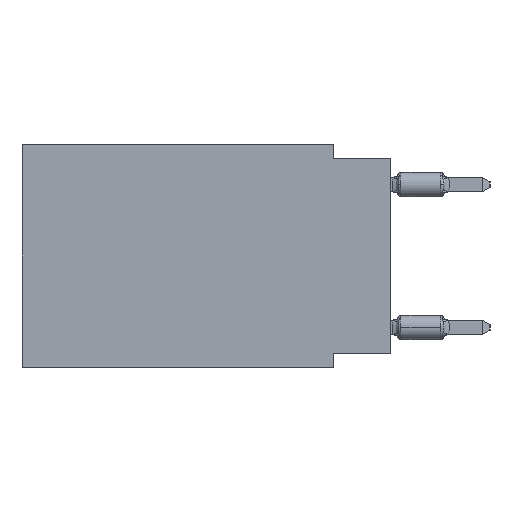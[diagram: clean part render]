
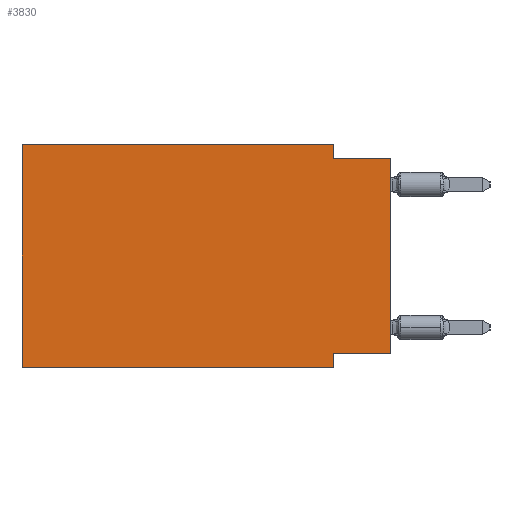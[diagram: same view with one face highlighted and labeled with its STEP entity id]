
A CAD part, left-side view. The second image highlights one B-rep face of the part: STEP entity #3830.
In plain terms, the highlighted planar face has unit normal (-1, 0, 0).
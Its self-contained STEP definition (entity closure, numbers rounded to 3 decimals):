
#360 = DIRECTION ( 'NONE',  ( 0., -1., 0. ) ) ;
#802 = EDGE_CURVE ( 'NONE', #33321, #27823, #25058, .T. ) ;
#835 = VECTOR ( 'NONE', #31269, 1000. ) ;
#912 = CARTESIAN_POINT ( 'NONE',  ( 0., 0., -9.271 ) ) ;
#1243 = VECTOR ( 'NONE', #7955, 1000. ) ;
#1660 = VERTEX_POINT ( 'NONE', #35047 ) ;
#2793 = CARTESIAN_POINT ( 'NONE',  ( 0., 0., 0. ) ) ;
#3195 = DIRECTION ( 'NONE',  ( 0., 0., -1. ) ) ;
#3286 = LINE ( 'NONE', #35207, #33391 ) ;
#3577 = CARTESIAN_POINT ( 'NONE',  ( 0., 0., -9.271 ) ) ;
#3830 = ADVANCED_FACE ( 'NONE', ( #6949 ), #16720, .F. ) ;
#3994 = VERTEX_POINT ( 'NONE', #18133 ) ;
#6949 = FACE_OUTER_BOUND ( 'NONE', #22570, .T. ) ;
#7066 = VERTEX_POINT ( 'NONE', #29626 ) ;
#7770 = EDGE_CURVE ( 'NONE', #33321, #39547, #39243, .T. ) ;
#7955 = DIRECTION ( 'NONE',  ( 0., 0., -1. ) ) ;
#9227 = DIRECTION ( 'NONE',  ( 0., 0., 1. ) ) ;
#9250 = EDGE_CURVE ( 'NONE', #3994, #37049, #32625, .T. ) ;
#9522 = ORIENTED_EDGE ( 'NONE', *, *, #7770, .F. ) ;
#10054 = CARTESIAN_POINT ( 'NONE',  ( 0., 16.383, 0. ) ) ;
#10236 = ORIENTED_EDGE ( 'NONE', *, *, #27374, .T. ) ;
#10710 = CARTESIAN_POINT ( 'NONE',  ( 0., 2.54, -0.635 ) ) ;
#11444 = VECTOR ( 'NONE', #3195, 1000. ) ;
#12144 = ORIENTED_EDGE ( 'NONE', *, *, #9250, .F. ) ;
#12606 = CARTESIAN_POINT ( 'NONE',  ( 0., 16.383, -9.906 ) ) ;
#12702 = ORIENTED_EDGE ( 'NONE', *, *, #802, .T. ) ;
#13578 = DIRECTION ( 'NONE',  ( 0., 1., 0. ) ) ;
#14728 = EDGE_CURVE ( 'NONE', #1660, #27823, #38011, .T. ) ;
#15054 = LINE ( 'NONE', #2793, #38530 ) ;
#15615 = CARTESIAN_POINT ( 'NONE',  ( 0., 2.54, -9.906 ) ) ;
#15654 = DIRECTION ( 'NONE',  ( 0., -1., 0. ) ) ;
#16720 = PLANE ( 'NONE',  #26188 ) ;
#18133 = CARTESIAN_POINT ( 'NONE',  ( 0., 2.54, 0. ) ) ;
#18554 = CARTESIAN_POINT ( 'NONE',  ( 0., 2.54, -9.906 ) ) ;
#20129 = ORIENTED_EDGE ( 'NONE', *, *, #39391, .F. ) ;
#20402 = DIRECTION ( 'NONE',  ( 0., 0., 1. ) ) ;
#20620 = VECTOR ( 'NONE', #15654, 1000. ) ;
#22570 = EDGE_LOOP ( 'NONE', ( #10236, #20129, #12144, #40866, #9522, #12702, #38331, #23306 ) ) ;
#23211 = VERTEX_POINT ( 'NONE', #3577 ) ;
#23306 = ORIENTED_EDGE ( 'NONE', *, *, #28640, .F. ) ;
#23527 = DIRECTION ( 'NONE',  ( 1., 0., 0. ) ) ;
#23925 = CARTESIAN_POINT ( 'NONE',  ( 0., 2.54, 0. ) ) ;
#23994 = CARTESIAN_POINT ( 'NONE',  ( 0., 16.383, 0. ) ) ;
#25058 = LINE ( 'NONE', #12606, #835 ) ;
#26188 = AXIS2_PLACEMENT_3D ( 'NONE', #10054, #23527, #36167 ) ;
#26202 = EDGE_CURVE ( 'NONE', #39547, #3994, #27674, .T. ) ;
#27124 = VECTOR ( 'NONE', #20402, 1000. ) ;
#27374 = EDGE_CURVE ( 'NONE', #23211, #7066, #15054, .T. ) ;
#27674 = LINE ( 'NONE', #37608, #20620 ) ;
#27823 = VERTEX_POINT ( 'NONE', #15615 ) ;
#28640 = EDGE_CURVE ( 'NONE', #23211, #1660, #29337, .T. ) ;
#29337 = LINE ( 'NONE', #912, #37965 ) ;
#29626 = CARTESIAN_POINT ( 'NONE',  ( 0., 0., -0.635 ) ) ;
#29890 = CARTESIAN_POINT ( 'NONE',  ( 0., 16.383, -9.906 ) ) ;
#31269 = DIRECTION ( 'NONE',  ( 0., -1., 0. ) ) ;
#32625 = LINE ( 'NONE', #23925, #1243 ) ;
#33321 = VERTEX_POINT ( 'NONE', #29890 ) ;
#33391 = VECTOR ( 'NONE', #360, 1000. ) ;
#35047 = CARTESIAN_POINT ( 'NONE',  ( 0., 2.54, -9.271 ) ) ;
#35207 = CARTESIAN_POINT ( 'NONE',  ( 0., 0., -0.635 ) ) ;
#36167 = DIRECTION ( 'NONE',  ( 0., 0., -1. ) ) ;
#37049 = VERTEX_POINT ( 'NONE', #10710 ) ;
#37608 = CARTESIAN_POINT ( 'NONE',  ( 0., 16.383, 0. ) ) ;
#37965 = VECTOR ( 'NONE', #13578, 1000. ) ;
#38011 = LINE ( 'NONE', #18554, #11444 ) ;
#38331 = ORIENTED_EDGE ( 'NONE', *, *, #14728, .F. ) ;
#38428 = CARTESIAN_POINT ( 'NONE',  ( 0., 16.383, 0. ) ) ;
#38530 = VECTOR ( 'NONE', #9227, 1000. ) ;
#39243 = LINE ( 'NONE', #38428, #27124 ) ;
#39391 = EDGE_CURVE ( 'NONE', #37049, #7066, #3286, .T. ) ;
#39547 = VERTEX_POINT ( 'NONE', #23994 ) ;
#40866 = ORIENTED_EDGE ( 'NONE', *, *, #26202, .F. ) ;
